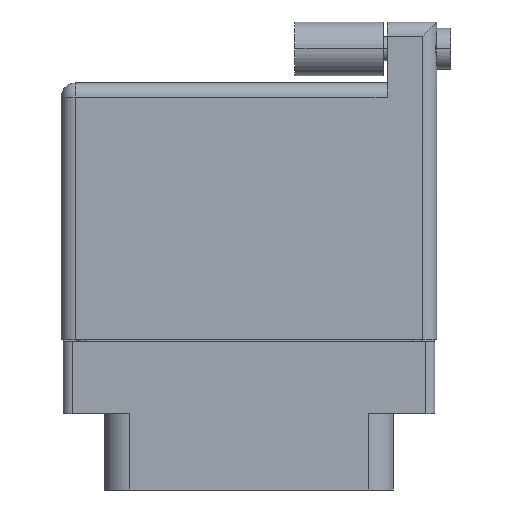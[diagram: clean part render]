
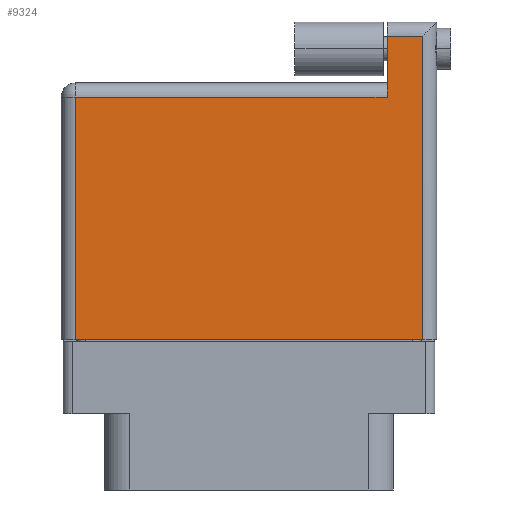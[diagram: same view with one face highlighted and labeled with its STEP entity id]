
A CAD part, front view. The second image highlights one B-rep face of the part: STEP entity #9324.
In plain terms, the highlighted face is planar.
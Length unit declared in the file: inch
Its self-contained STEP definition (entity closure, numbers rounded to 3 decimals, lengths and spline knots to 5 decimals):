
#338 = ORIENTED_EDGE ( 'NONE', *, *, #8909, .T. ) ;
#1061 = VECTOR ( 'NONE', #17739, 39.37008 ) ;
#1391 = CARTESIAN_POINT ( 'NONE',  ( -0.6125, 0.756, 0.3575 ) ) ;
#1940 = AXIS2_PLACEMENT_3D ( 'NONE', #6362, #16810, #13559 ) ;
#2232 = VERTEX_POINT ( 'NONE', #14613 ) ;
#2894 = CARTESIAN_POINT ( 'NONE',  ( 0.6125, 0.97, 0.3575 ) ) ;
#3079 = EDGE_CURVE ( 'NONE', #6696, #2232, #15630, .T. ) ;
#3089 = ORIENTED_EDGE ( 'NONE', *, *, #13420, .T. ) ;
#3419 = CARTESIAN_POINT ( 'NONE',  ( -0.6625, -0.1, 0.3575 ) ) ;
#3518 = ORIENTED_EDGE ( 'NONE', *, *, #21688, .T. ) ;
#5196 = CARTESIAN_POINT ( 'NONE',  ( 0.4875, 1.02, 0.3575 ) ) ;
#6362 = CARTESIAN_POINT ( 'NONE',  ( -0.6625, 0.806, 0.3575 ) ) ;
#6367 = CARTESIAN_POINT ( 'NONE',  ( -0.6125, -0.1, 0.3575 ) ) ;
#6696 = VERTEX_POINT ( 'NONE', #2894 ) ;
#7582 = VERTEX_POINT ( 'NONE', #6367 ) ;
#7626 = VECTOR ( 'NONE', #10414, 39.37008 ) ;
#8909 = EDGE_CURVE ( 'NONE', #7582, #19646, #16719, .T. ) ;
#9324 = ADVANCED_FACE ( 'NONE', ( #18378 ), #11778, .F. ) ;
#9781 = VECTOR ( 'NONE', #19045, 39.37008 ) ;
#9899 = VECTOR ( 'NONE', #19991, 39.37008 ) ;
#9904 = ORIENTED_EDGE ( 'NONE', *, *, #3079, .T. ) ;
#10414 = DIRECTION ( 'NONE',  ( 1., 0., 0. ) ) ;
#10474 = ORIENTED_EDGE ( 'NONE', *, *, #14240, .T. ) ;
#11061 = ORIENTED_EDGE ( 'NONE', *, *, #21626, .T. ) ;
#11152 = CARTESIAN_POINT ( 'NONE',  ( -0.6625, 0.756, 0.3575 ) ) ;
#11778 = PLANE ( 'NONE',  #1940 ) ;
#13093 = LINE ( 'NONE', #5196, #9781 ) ;
#13222 = LINE ( 'NONE', #11152, #9899 ) ;
#13420 = EDGE_CURVE ( 'NONE', #21346, #19616, #13222, .T. ) ;
#13456 = CARTESIAN_POINT ( 'NONE',  ( -0.6125, -0.1, 0.3575 ) ) ;
#13559 = DIRECTION ( 'NONE',  ( -1., 0., 0. ) ) ;
#13649 = CARTESIAN_POINT ( 'NONE',  ( 0.6125, -0.1, 0.3575 ) ) ;
#13709 = CARTESIAN_POINT ( 'NONE',  ( 0.6125, 1.02, 0.3575 ) ) ;
#14240 = EDGE_CURVE ( 'NONE', #19616, #7582, #21965, .T. ) ;
#14465 = VECTOR ( 'NONE', #18817, 39.37008 ) ;
#14613 = CARTESIAN_POINT ( 'NONE',  ( 0.4875, 0.97, 0.3575 ) ) ;
#15630 = LINE ( 'NONE', #19437, #1061 ) ;
#16691 = LINE ( 'NONE', #13709, #22241 ) ;
#16719 = LINE ( 'NONE', #3419, #7626 ) ;
#16810 = DIRECTION ( 'NONE',  ( 0., 0., -1. ) ) ;
#17420 = DIRECTION ( 'NONE',  ( 0., 1., 0. ) ) ;
#17739 = DIRECTION ( 'NONE',  ( -1., 0., 0. ) ) ;
#18378 = FACE_OUTER_BOUND ( 'NONE', #18811, .T. ) ;
#18811 = EDGE_LOOP ( 'NONE', ( #338, #11061, #9904, #3518, #3089, #10474 ) ) ;
#18817 = DIRECTION ( 'NONE',  ( 0., -1., 0. ) ) ;
#19045 = DIRECTION ( 'NONE',  ( 0., -1., 0. ) ) ;
#19437 = CARTESIAN_POINT ( 'NONE',  ( -0.6625, 0.97, 0.3575 ) ) ;
#19616 = VERTEX_POINT ( 'NONE', #1391 ) ;
#19646 = VERTEX_POINT ( 'NONE', #13649 ) ;
#19899 = CARTESIAN_POINT ( 'NONE',  ( 0.4875, 0.756, 0.3575 ) ) ;
#19991 = DIRECTION ( 'NONE',  ( -1., 0., 0. ) ) ;
#21346 = VERTEX_POINT ( 'NONE', #19899 ) ;
#21626 = EDGE_CURVE ( 'NONE', #19646, #6696, #16691, .T. ) ;
#21688 = EDGE_CURVE ( 'NONE', #2232, #21346, #13093, .T. ) ;
#21965 = LINE ( 'NONE', #13456, #14465 ) ;
#22241 = VECTOR ( 'NONE', #17420, 39.37008 ) ;
